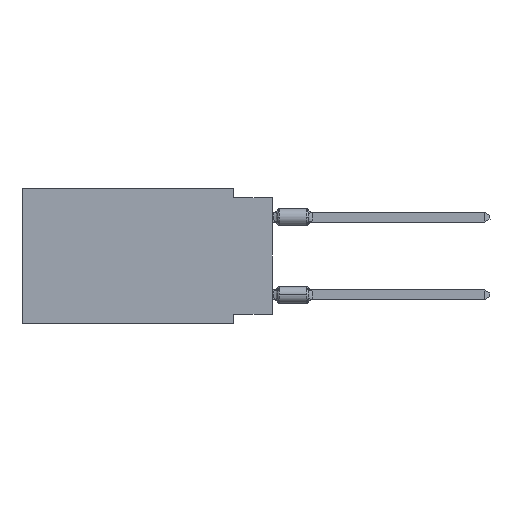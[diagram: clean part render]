
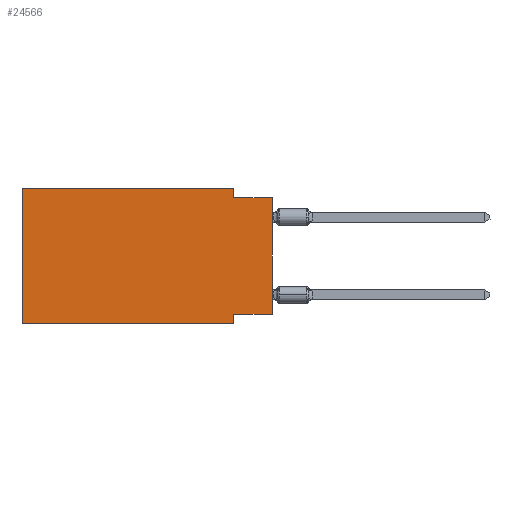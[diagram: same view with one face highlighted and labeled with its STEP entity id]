
A CAD part, left-side view. The second image highlights one B-rep face of the part: STEP entity #24566.
In plain terms, the highlighted planar face has unit normal (-1, 0, 0).
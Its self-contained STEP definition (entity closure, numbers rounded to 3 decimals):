
#366 = VERTEX_POINT ( 'NONE', #20620 ) ;
#388 = VECTOR ( 'NONE', #4768, 1000. ) ;
#656 = CARTESIAN_POINT ( 'NONE',  ( 0., 2.54, 0. ) ) ;
#1117 = DIRECTION ( 'NONE',  ( 0., -1., 0. ) ) ;
#1241 = AXIS2_PLACEMENT_3D ( 'NONE', #22614, #5768, #20670 ) ;
#1250 = CARTESIAN_POINT ( 'NONE',  ( 0., 2.54, -0.635 ) ) ;
#1509 = EDGE_CURVE ( 'NONE', #25479, #3943, #9398, .T. ) ;
#1744 = LINE ( 'NONE', #23324, #4202 ) ;
#2717 = EDGE_CURVE ( 'NONE', #25479, #31228, #19008, .T. ) ;
#2880 = VECTOR ( 'NONE', #19119, 1000. ) ;
#3943 = VERTEX_POINT ( 'NONE', #6699 ) ;
#4202 = VECTOR ( 'NONE', #1117, 1000. ) ;
#4538 = CARTESIAN_POINT ( 'NONE',  ( 0., 0., 0. ) ) ;
#4704 = EDGE_CURVE ( 'NONE', #18348, #21157, #22856, .T. ) ;
#4768 = DIRECTION ( 'NONE',  ( 0., 0., -1. ) ) ;
#4943 = DIRECTION ( 'NONE',  ( 0., -1., 0. ) ) ;
#5134 = CARTESIAN_POINT ( 'NONE',  ( 0., 2.54, -8.89 ) ) ;
#5768 = DIRECTION ( 'NONE',  ( 1., 0., 0. ) ) ;
#6699 = CARTESIAN_POINT ( 'NONE',  ( 0., 0., -0.635 ) ) ;
#6879 = CARTESIAN_POINT ( 'NONE',  ( 0., 16.383, -8.89 ) ) ;
#7093 = EDGE_CURVE ( 'NONE', #24152, #366, #24848, .T. ) ;
#7399 = VECTOR ( 'NONE', #9048, 1000. ) ;
#8322 = EDGE_CURVE ( 'NONE', #31228, #17480, #11898, .T. ) ;
#8742 = LINE ( 'NONE', #23637, #7399 ) ;
#8815 = CARTESIAN_POINT ( 'NONE',  ( 0., 0., -8.255 ) ) ;
#9048 = DIRECTION ( 'NONE',  ( 0., -1., 0. ) ) ;
#9398 = LINE ( 'NONE', #4538, #2880 ) ;
#9596 = ORIENTED_EDGE ( 'NONE', *, *, #7093, .F. ) ;
#9775 = CARTESIAN_POINT ( 'NONE',  ( 0., 16.383, 0. ) ) ;
#10161 = VECTOR ( 'NONE', #16744, 1000. ) ;
#11006 = ORIENTED_EDGE ( 'NONE', *, *, #2717, .F. ) ;
#11898 = LINE ( 'NONE', #24201, #388 ) ;
#12172 = ORIENTED_EDGE ( 'NONE', *, *, #8322, .F. ) ;
#12211 = VECTOR ( 'NONE', #18006, 1000. ) ;
#12257 = FACE_OUTER_BOUND ( 'NONE', #18781, .T. ) ;
#14094 = EDGE_CURVE ( 'NONE', #24152, #17480, #1744, .T. ) ;
#14742 = ORIENTED_EDGE ( 'NONE', *, *, #15212, .F. ) ;
#14778 = EDGE_CURVE ( 'NONE', #366, #18348, #19843, .T. ) ;
#15212 = EDGE_CURVE ( 'NONE', #21157, #3943, #8742, .T. ) ;
#16707 = VECTOR ( 'NONE', #4943, 1000. ) ;
#16744 = DIRECTION ( 'NONE',  ( 0., 1., 0. ) ) ;
#17271 = ORIENTED_EDGE ( 'NONE', *, *, #14094, .T. ) ;
#17480 = VERTEX_POINT ( 'NONE', #5134 ) ;
#17562 = DIRECTION ( 'NONE',  ( 0., 0., 1. ) ) ;
#18006 = DIRECTION ( 'NONE',  ( 0., 0., -1. ) ) ;
#18092 = PLANE ( 'NONE',  #1241 ) ;
#18348 = VERTEX_POINT ( 'NONE', #20725 ) ;
#18781 = EDGE_LOOP ( 'NONE', ( #23958, #14742, #28068, #19896, #9596, #17271, #12172, #11006 ) ) ;
#19008 = LINE ( 'NONE', #8815, #10161 ) ;
#19119 = DIRECTION ( 'NONE',  ( 0., 0., 1. ) ) ;
#19843 = LINE ( 'NONE', #27154, #16707 ) ;
#19896 = ORIENTED_EDGE ( 'NONE', *, *, #14778, .F. ) ;
#20620 = CARTESIAN_POINT ( 'NONE',  ( 0., 16.383, 0. ) ) ;
#20670 = DIRECTION ( 'NONE',  ( 0., 0., -1. ) ) ;
#20725 = CARTESIAN_POINT ( 'NONE',  ( 0., 2.54, 0. ) ) ;
#21157 = VERTEX_POINT ( 'NONE', #1250 ) ;
#21526 = VECTOR ( 'NONE', #17562, 1000. ) ;
#22614 = CARTESIAN_POINT ( 'NONE',  ( 0., 16.383, 0. ) ) ;
#22856 = LINE ( 'NONE', #656, #12211 ) ;
#23324 = CARTESIAN_POINT ( 'NONE',  ( 0., 16.383, -8.89 ) ) ;
#23637 = CARTESIAN_POINT ( 'NONE',  ( 0., 0., -0.635 ) ) ;
#23958 = ORIENTED_EDGE ( 'NONE', *, *, #1509, .T. ) ;
#24152 = VERTEX_POINT ( 'NONE', #6879 ) ;
#24201 = CARTESIAN_POINT ( 'NONE',  ( 0., 2.54, -8.89 ) ) ;
#24566 = ADVANCED_FACE ( 'NONE', ( #12257 ), #18092, .F. ) ;
#24848 = LINE ( 'NONE', #9775, #21526 ) ;
#25479 = VERTEX_POINT ( 'NONE', #27101 ) ;
#27101 = CARTESIAN_POINT ( 'NONE',  ( 0., 0., -8.255 ) ) ;
#27154 = CARTESIAN_POINT ( 'NONE',  ( 0., 16.383, 0. ) ) ;
#28068 = ORIENTED_EDGE ( 'NONE', *, *, #4704, .F. ) ;
#28648 = CARTESIAN_POINT ( 'NONE',  ( 0., 2.54, -8.255 ) ) ;
#31228 = VERTEX_POINT ( 'NONE', #28648 ) ;
